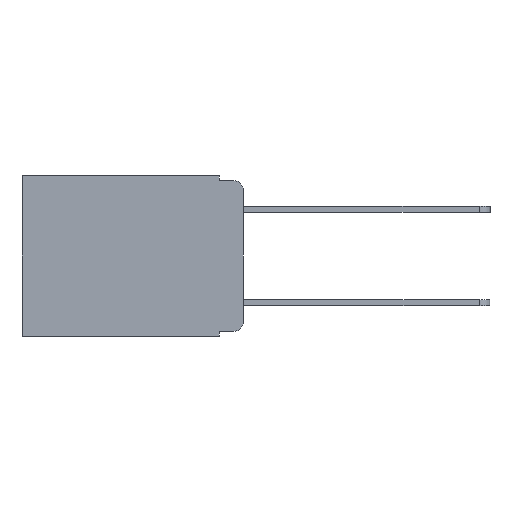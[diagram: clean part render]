
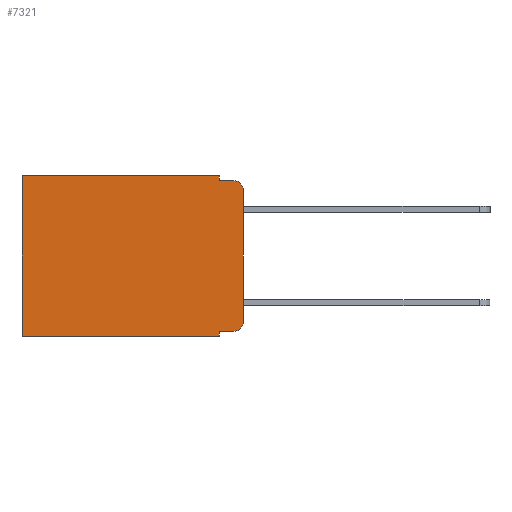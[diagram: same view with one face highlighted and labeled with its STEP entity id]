
A CAD part, left-side view. The second image highlights one B-rep face of the part: STEP entity #7321.
In plain terms, the highlighted planar face has unit normal (-1, 0, 0).
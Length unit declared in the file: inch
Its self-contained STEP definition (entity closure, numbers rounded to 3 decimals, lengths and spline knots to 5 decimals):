
#199 = EDGE_CURVE ( 'NONE', #1981, #4881, #4358, .T. ) ;
#250 = VERTEX_POINT ( 'NONE', #3866 ) ;
#284 = VERTEX_POINT ( 'NONE', #5289 ) ;
#320 = VERTEX_POINT ( 'NONE', #5108 ) ;
#377 = CARTESIAN_POINT ( 'NONE',  ( 0.298, 0., -0.343 ) ) ;
#399 = ORIENTED_EDGE ( 'NONE', *, *, #199, .T. ) ;
#605 = DIRECTION ( 'NONE',  ( 0., 0., -1. ) ) ;
#614 = ORIENTED_EDGE ( 'NONE', *, *, #8945, .F. ) ;
#690 = DIRECTION ( 'NONE',  ( 0., -1., 0. ) ) ;
#821 = VECTOR ( 'NONE', #5937, 39.37008 ) ;
#892 = ORIENTED_EDGE ( 'NONE', *, *, #4355, .T. ) ;
#1283 = CARTESIAN_POINT ( 'NONE',  ( 0.298, 0.051, 0. ) ) ;
#1378 = CIRCLE ( 'NONE', #8743, 0.02 ) ;
#1505 = ORIENTED_EDGE ( 'NONE', *, *, #2111, .F. ) ;
#1866 = EDGE_CURVE ( 'NONE', #1981, #4647, #7040, .T. ) ;
#1892 = CARTESIAN_POINT ( 'NONE',  ( 0.298, 0.473, 0. ) ) ;
#1893 = ORIENTED_EDGE ( 'NONE', *, *, #6292, .T. ) ;
#1908 = CARTESIAN_POINT ( 'NONE',  ( 0.298, 0.051, -0.343 ) ) ;
#1981 = VERTEX_POINT ( 'NONE', #8720 ) ;
#2111 = EDGE_CURVE ( 'NONE', #4647, #284, #5342, .T. ) ;
#2115 = ORIENTED_EDGE ( 'NONE', *, *, #3888, .F. ) ;
#2245 = ORIENTED_EDGE ( 'NONE', *, *, #7655, .F. ) ;
#2408 = VECTOR ( 'NONE', #5933, 39.37008 ) ;
#2606 = ORIENTED_EDGE ( 'NONE', *, *, #6838, .T. ) ;
#2738 = CIRCLE ( 'NONE', #4202, 0.02 ) ;
#2832 = VERTEX_POINT ( 'NONE', #1892 ) ;
#2996 = CARTESIAN_POINT ( 'NONE',  ( 0.298, 0.02, -0.333 ) ) ;
#3205 = VECTOR ( 'NONE', #6036, 39.37008 ) ;
#3218 = PLANE ( 'NONE',  #6239 ) ;
#3297 = FACE_OUTER_BOUND ( 'NONE', #4772, .T. ) ;
#3355 = DIRECTION ( 'NONE',  ( 0., 0., -1. ) ) ;
#3514 = DIRECTION ( 'NONE',  ( 0., 0., -1. ) ) ;
#3684 = DIRECTION ( 'NONE',  ( -1., 0., 0. ) ) ;
#3742 = LINE ( 'NONE', #8369, #5202 ) ;
#3866 = CARTESIAN_POINT ( 'NONE',  ( 0.298, 0., -0.03 ) ) ;
#3888 = EDGE_CURVE ( 'NONE', #7750, #320, #7667, .T. ) ;
#3957 = DIRECTION ( 'NONE',  ( 0., 0., -1. ) ) ;
#4097 = CARTESIAN_POINT ( 'NONE',  ( 0.298, 0.02, -0.03 ) ) ;
#4202 = AXIS2_PLACEMENT_3D ( 'NONE', #4097, #8731, #4815 ) ;
#4355 = EDGE_CURVE ( 'NONE', #8492, #2832, #4832, .T. ) ;
#4358 = LINE ( 'NONE', #5973, #2408 ) ;
#4430 = ORIENTED_EDGE ( 'NONE', *, *, #1866, .F. ) ;
#4619 = VECTOR ( 'NONE', #3355, 39.37008 ) ;
#4647 = VERTEX_POINT ( 'NONE', #1908 ) ;
#4772 = EDGE_LOOP ( 'NONE', ( #614, #1893, #2115, #2245, #892, #2606, #1505, #4430, #399, #6595 ) ) ;
#4815 = DIRECTION ( 'NONE',  ( 0., 0., -1. ) ) ;
#4832 = LINE ( 'NONE', #6609, #821 ) ;
#4845 = LINE ( 'NONE', #6160, #4619 ) ;
#4881 = VERTEX_POINT ( 'NONE', #2996 ) ;
#5108 = CARTESIAN_POINT ( 'NONE',  ( 0.298, 0.02, -0.01 ) ) ;
#5202 = VECTOR ( 'NONE', #605, 39.37008 ) ;
#5289 = CARTESIAN_POINT ( 'NONE',  ( 0.298, 0.473, -0.343 ) ) ;
#5342 = LINE ( 'NONE', #377, #3205 ) ;
#5914 = CARTESIAN_POINT ( 'NONE',  ( 0.298, 0.051, -0.01 ) ) ;
#5926 = VECTOR ( 'NONE', #690, 39.37008 ) ;
#5933 = DIRECTION ( 'NONE',  ( 0., -1., 0. ) ) ;
#5937 = DIRECTION ( 'NONE',  ( 0., 1., 0. ) ) ;
#5973 = CARTESIAN_POINT ( 'NONE',  ( 0.298, 0.051, -0.333 ) ) ;
#6036 = DIRECTION ( 'NONE',  ( 0., 1., 0. ) ) ;
#6079 = CARTESIAN_POINT ( 'NONE',  ( 0.298, 0.473, 0. ) ) ;
#6160 = CARTESIAN_POINT ( 'NONE',  ( 0.298, 0., 0. ) ) ;
#6239 = AXIS2_PLACEMENT_3D ( 'NONE', #7378, #7974, #3957 ) ;
#6292 = EDGE_CURVE ( 'NONE', #250, #320, #2738, .T. ) ;
#6595 = ORIENTED_EDGE ( 'NONE', *, *, #8095, .T. ) ;
#6609 = CARTESIAN_POINT ( 'NONE',  ( 0.298, 0., 0. ) ) ;
#6637 = CARTESIAN_POINT ( 'NONE',  ( 0.298, 0., -0.313 ) ) ;
#6729 = VERTEX_POINT ( 'NONE', #6637 ) ;
#6838 = EDGE_CURVE ( 'NONE', #2832, #284, #7228, .T. ) ;
#6928 = CARTESIAN_POINT ( 'NONE',  ( 0.298, 0.051, 0. ) ) ;
#7040 = LINE ( 'NONE', #1283, #8692 ) ;
#7228 = LINE ( 'NONE', #6079, #8672 ) ;
#7321 = ADVANCED_FACE ( 'NONE', ( #3297 ), #3218, .F. ) ;
#7378 = CARTESIAN_POINT ( 'NONE',  ( 0.298, 0., 0. ) ) ;
#7411 = DIRECTION ( 'NONE',  ( 0., 0., -1. ) ) ;
#7655 = EDGE_CURVE ( 'NONE', #8492, #7750, #3742, .T. ) ;
#7667 = LINE ( 'NONE', #7855, #5926 ) ;
#7750 = VERTEX_POINT ( 'NONE', #5914 ) ;
#7757 = CARTESIAN_POINT ( 'NONE',  ( 0.298, 0.02, -0.313 ) ) ;
#7855 = CARTESIAN_POINT ( 'NONE',  ( 0.298, 0.051, -0.01 ) ) ;
#7974 = DIRECTION ( 'NONE',  ( 1., 0., 0. ) ) ;
#8095 = EDGE_CURVE ( 'NONE', #4881, #6729, #1378, .T. ) ;
#8362 = DIRECTION ( 'NONE',  ( 0., 0., -1. ) ) ;
#8369 = CARTESIAN_POINT ( 'NONE',  ( 0.298, 0.051, 0. ) ) ;
#8492 = VERTEX_POINT ( 'NONE', #6928 ) ;
#8672 = VECTOR ( 'NONE', #7411, 39.37008 ) ;
#8692 = VECTOR ( 'NONE', #3514, 39.37008 ) ;
#8720 = CARTESIAN_POINT ( 'NONE',  ( 0.298, 0.051, -0.333 ) ) ;
#8731 = DIRECTION ( 'NONE',  ( -1., 0., 0. ) ) ;
#8743 = AXIS2_PLACEMENT_3D ( 'NONE', #7757, #3684, #8362 ) ;
#8945 = EDGE_CURVE ( 'NONE', #250, #6729, #4845, .T. ) ;
